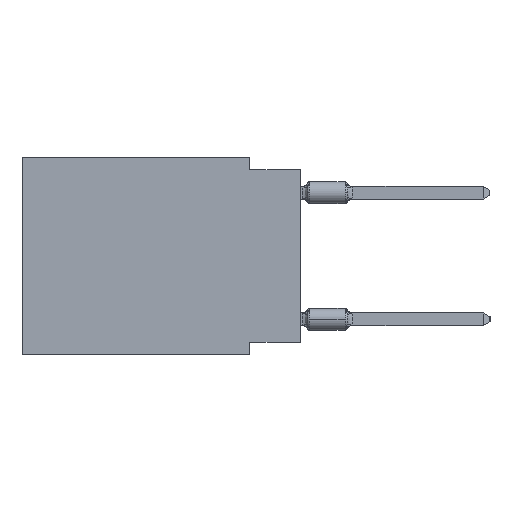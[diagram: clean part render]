
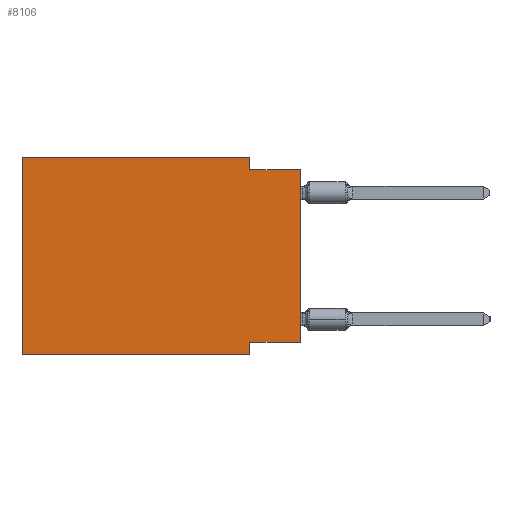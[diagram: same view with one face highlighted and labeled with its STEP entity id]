
A CAD part, left-side view. The second image highlights one B-rep face of the part: STEP entity #8106.
In plain terms, the highlighted planar face has unit normal (-1, 0, 0).
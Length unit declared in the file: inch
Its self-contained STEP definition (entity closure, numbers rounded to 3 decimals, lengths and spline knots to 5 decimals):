
#182 = ORIENTED_EDGE ( 'NONE', *, *, #15636, .T. ) ;
#710 = CARTESIAN_POINT ( 'NONE',  ( 0., 0.1, -0.365 ) ) ;
#1048 = CARTESIAN_POINT ( 'NONE',  ( 0., 0.1, -0.39 ) ) ;
#1149 = VECTOR ( 'NONE', #20828, 39.37008 ) ;
#1955 = DIRECTION ( 'NONE',  ( 0., -1., 0. ) ) ;
#2383 = CARTESIAN_POINT ( 'NONE',  ( 0., 0.55, 0. ) ) ;
#2669 = DIRECTION ( 'NONE',  ( 0., 1., 0. ) ) ;
#3692 = LINE ( 'NONE', #10103, #1149 ) ;
#5462 = CARTESIAN_POINT ( 'NONE',  ( 0., 0.1, -0.39 ) ) ;
#5611 = CARTESIAN_POINT ( 'NONE',  ( 0., 0.55, -0.39 ) ) ;
#6040 = VECTOR ( 'NONE', #2669, 39.37008 ) ;
#7689 = VERTEX_POINT ( 'NONE', #29480 ) ;
#8106 = ADVANCED_FACE ( 'NONE', ( #29825 ), #43780, .F. ) ;
#8631 = DIRECTION ( 'NONE',  ( 0., -1., 0. ) ) ;
#8685 = DIRECTION ( 'NONE',  ( 0., 0., 1. ) ) ;
#10103 = CARTESIAN_POINT ( 'NONE',  ( 0., 0., -0.025 ) ) ;
#10197 = VERTEX_POINT ( 'NONE', #18902 ) ;
#10233 = EDGE_CURVE ( 'NONE', #36582, #10197, #30083, .T. ) ;
#10636 = VECTOR ( 'NONE', #14983, 39.37008 ) ;
#11115 = ORIENTED_EDGE ( 'NONE', *, *, #20422, .F. ) ;
#11282 = CARTESIAN_POINT ( 'NONE',  ( 0., 0., 0. ) ) ;
#12451 = DIRECTION ( 'NONE',  ( 1., 0., 0. ) ) ;
#12622 = VECTOR ( 'NONE', #25215, 39.37008 ) ;
#12998 = VECTOR ( 'NONE', #36964, 39.37008 ) ;
#13824 = ORIENTED_EDGE ( 'NONE', *, *, #44783, .F. ) ;
#14983 = DIRECTION ( 'NONE',  ( 0., 0., -1. ) ) ;
#15636 = EDGE_CURVE ( 'NONE', #7689, #18072, #33269, .T. ) ;
#15869 = EDGE_CURVE ( 'NONE', #26508, #24354, #25678, .T. ) ;
#17113 = VECTOR ( 'NONE', #8685, 39.37008 ) ;
#18072 = VERTEX_POINT ( 'NONE', #5462 ) ;
#18902 = CARTESIAN_POINT ( 'NONE',  ( 0., 0.1, -0.025 ) ) ;
#19786 = CARTESIAN_POINT ( 'NONE',  ( 0., 0.1, 0. ) ) ;
#20157 = ORIENTED_EDGE ( 'NONE', *, *, #15869, .T. ) ;
#20422 = EDGE_CURVE ( 'NONE', #7689, #24296, #38881, .T. ) ;
#20828 = DIRECTION ( 'NONE',  ( 0., -1., 0. ) ) ;
#23069 = CARTESIAN_POINT ( 'NONE',  ( 0., 0.1, 0. ) ) ;
#24296 = VERTEX_POINT ( 'NONE', #25222 ) ;
#24354 = VERTEX_POINT ( 'NONE', #30396 ) ;
#24901 = VECTOR ( 'NONE', #1955, 39.37008 ) ;
#25082 = VECTOR ( 'NONE', #8631, 39.37008 ) ;
#25215 = DIRECTION ( 'NONE',  ( 0., 0., 1. ) ) ;
#25222 = CARTESIAN_POINT ( 'NONE',  ( 0., 0.55, 0. ) ) ;
#25665 = EDGE_CURVE ( 'NONE', #10197, #24354, #3692, .T. ) ;
#25678 = LINE ( 'NONE', #11282, #12622 ) ;
#25812 = CARTESIAN_POINT ( 'NONE',  ( 0., 0.55, 0. ) ) ;
#25904 = VERTEX_POINT ( 'NONE', #710 ) ;
#25979 = LINE ( 'NONE', #36524, #25082 ) ;
#26375 = DIRECTION ( 'NONE',  ( 0., 0., -1. ) ) ;
#26508 = VERTEX_POINT ( 'NONE', #34625 ) ;
#28748 = ORIENTED_EDGE ( 'NONE', *, *, #10233, .F. ) ;
#29480 = CARTESIAN_POINT ( 'NONE',  ( 0., 0.55, -0.39 ) ) ;
#29825 = FACE_OUTER_BOUND ( 'NONE', #33511, .T. ) ;
#30083 = LINE ( 'NONE', #19786, #12998 ) ;
#30396 = CARTESIAN_POINT ( 'NONE',  ( 0., 0., -0.025 ) ) ;
#32378 = LINE ( 'NONE', #1048, #10636 ) ;
#33141 = ORIENTED_EDGE ( 'NONE', *, *, #39863, .F. ) ;
#33269 = LINE ( 'NONE', #5611, #24901 ) ;
#33511 = EDGE_LOOP ( 'NONE', ( #20157, #38480, #28748, #44816, #11115, #182, #13824, #33141 ) ) ;
#33987 = LINE ( 'NONE', #40651, #6040 ) ;
#34625 = CARTESIAN_POINT ( 'NONE',  ( 0., 0., -0.365 ) ) ;
#34940 = AXIS2_PLACEMENT_3D ( 'NONE', #2383, #12451, #26375 ) ;
#36524 = CARTESIAN_POINT ( 'NONE',  ( 0., 0.55, 0. ) ) ;
#36582 = VERTEX_POINT ( 'NONE', #23069 ) ;
#36964 = DIRECTION ( 'NONE',  ( 0., 0., -1. ) ) ;
#38480 = ORIENTED_EDGE ( 'NONE', *, *, #25665, .F. ) ;
#38881 = LINE ( 'NONE', #25812, #17113 ) ;
#39863 = EDGE_CURVE ( 'NONE', #26508, #25904, #33987, .T. ) ;
#40651 = CARTESIAN_POINT ( 'NONE',  ( 0., 0., -0.365 ) ) ;
#40912 = EDGE_CURVE ( 'NONE', #24296, #36582, #25979, .T. ) ;
#43780 = PLANE ( 'NONE',  #34940 ) ;
#44783 = EDGE_CURVE ( 'NONE', #25904, #18072, #32378, .T. ) ;
#44816 = ORIENTED_EDGE ( 'NONE', *, *, #40912, .F. ) ;
